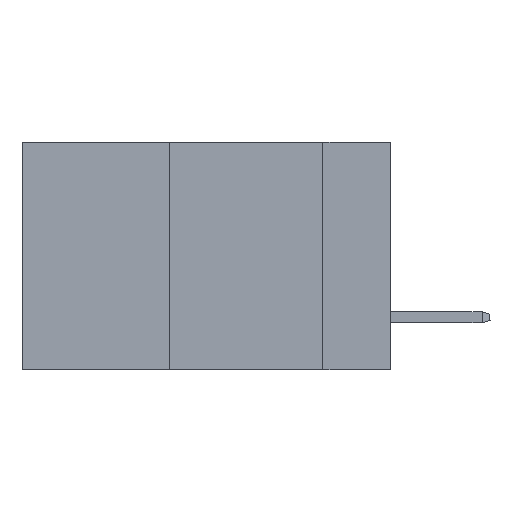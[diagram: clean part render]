
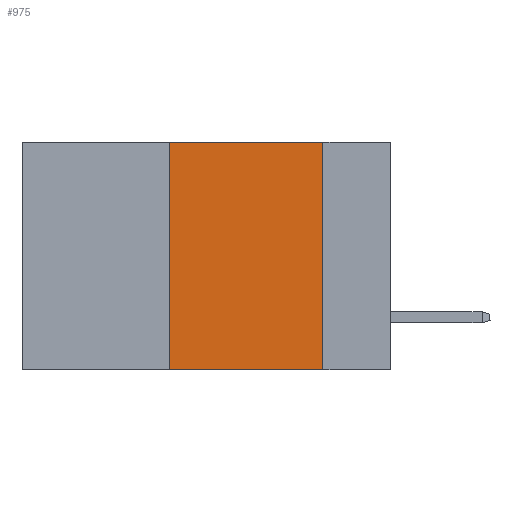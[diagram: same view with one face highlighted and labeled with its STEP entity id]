
A CAD part, left-side view. The second image highlights one B-rep face of the part: STEP entity #975.
In plain terms, the highlighted planar face has unit normal (-1, 0, 0).
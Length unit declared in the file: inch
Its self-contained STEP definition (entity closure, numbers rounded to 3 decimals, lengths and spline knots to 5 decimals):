
#225 = DIRECTION ( 'NONE',  ( 0., 0., -1. ) ) ;
#495 = ORIENTED_EDGE ( 'NONE', *, *, #9206, .F. ) ;
#783 = DIRECTION ( 'NONE',  ( 0., 0., 1. ) ) ;
#911 = ORIENTED_EDGE ( 'NONE', *, *, #2187, .F. ) ;
#939 = CARTESIAN_POINT ( 'NONE',  ( 0., 0.36, -0.37 ) ) ;
#975 = ADVANCED_FACE ( 'NONE', ( #3955 ), #4593, .F. ) ;
#1362 = EDGE_LOOP ( 'NONE', ( #911, #495, #7102, #7823 ) ) ;
#2093 = VECTOR ( 'NONE', #783, 39.37008 ) ;
#2187 = EDGE_CURVE ( 'NONE', #3411, #11251, #10880, .T. ) ;
#2275 = DIRECTION ( 'NONE',  ( 0., -1., 0. ) ) ;
#2972 = CARTESIAN_POINT ( 'NONE',  ( 0., 0.11, 0. ) ) ;
#3411 = VERTEX_POINT ( 'NONE', #2972 ) ;
#3681 = CARTESIAN_POINT ( 'NONE',  ( 0., 0.6, 0. ) ) ;
#3955 = FACE_OUTER_BOUND ( 'NONE', #1362, .T. ) ;
#4061 = LINE ( 'NONE', #6809, #11152 ) ;
#4593 = PLANE ( 'NONE',  #8105 ) ;
#5230 = CARTESIAN_POINT ( 'NONE',  ( 0., 0.36, 0. ) ) ;
#5640 = VERTEX_POINT ( 'NONE', #7508 ) ;
#6372 = DIRECTION ( 'NONE',  ( 1., 0., 0. ) ) ;
#6395 = VERTEX_POINT ( 'NONE', #939 ) ;
#6746 = CARTESIAN_POINT ( 'NONE',  ( 0., 0.6, -0.37 ) ) ;
#6809 = CARTESIAN_POINT ( 'NONE',  ( 0., 0.6, 0. ) ) ;
#6885 = DIRECTION ( 'NONE',  ( 0., 0., -1. ) ) ;
#7102 = ORIENTED_EDGE ( 'NONE', *, *, #9314, .F. ) ;
#7208 = LINE ( 'NONE', #6746, #8706 ) ;
#7508 = CARTESIAN_POINT ( 'NONE',  ( 0., 0.36, 0. ) ) ;
#7618 = DIRECTION ( 'NONE',  ( 0., -1., 0. ) ) ;
#7725 = CARTESIAN_POINT ( 'NONE',  ( 0., 0.11, 0. ) ) ;
#7823 = ORIENTED_EDGE ( 'NONE', *, *, #10346, .T. ) ;
#8011 = VECTOR ( 'NONE', #6885, 39.37008 ) ;
#8105 = AXIS2_PLACEMENT_3D ( 'NONE', #3681, #6372, #225 ) ;
#8706 = VECTOR ( 'NONE', #2275, 39.37008 ) ;
#9206 = EDGE_CURVE ( 'NONE', #5640, #3411, #4061, .T. ) ;
#9314 = EDGE_CURVE ( 'NONE', #6395, #5640, #10591, .T. ) ;
#9934 = CARTESIAN_POINT ( 'NONE',  ( 0., 0.11, -0.37 ) ) ;
#10346 = EDGE_CURVE ( 'NONE', #6395, #11251, #7208, .T. ) ;
#10591 = LINE ( 'NONE', #5230, #2093 ) ;
#10880 = LINE ( 'NONE', #7725, #8011 ) ;
#11152 = VECTOR ( 'NONE', #7618, 39.37008 ) ;
#11251 = VERTEX_POINT ( 'NONE', #9934 ) ;
